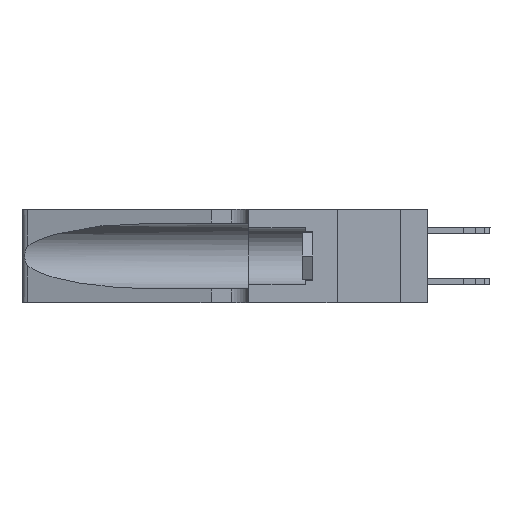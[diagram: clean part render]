
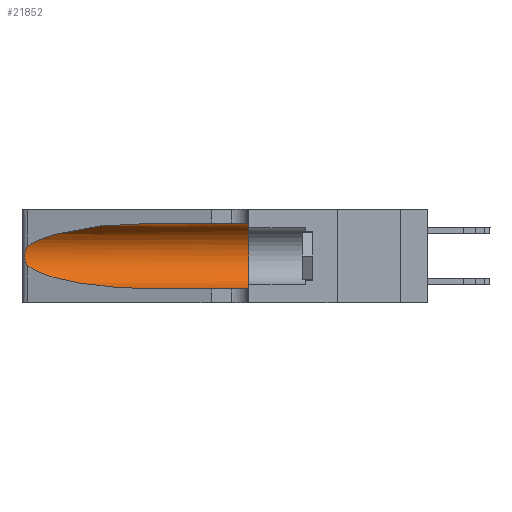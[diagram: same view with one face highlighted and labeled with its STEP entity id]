
A CAD part, left-side view. The second image highlights one B-rep face of the part: STEP entity #21852.
In plain terms, the highlighted cylindrical face has radius 3.308 mm (diameter 6.617 mm), a partial arc.
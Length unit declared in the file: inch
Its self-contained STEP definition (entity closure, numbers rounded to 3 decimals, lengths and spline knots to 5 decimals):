
#218 = CARTESIAN_POINT ( 'NONE',  ( 0.25487, 1.22718, 0.22369 ) ) ;
#322 = DIRECTION ( 'NONE',  ( 0., 0., 1. ) ) ;
#505 = ORIENTED_EDGE ( 'NONE', *, *, #8065, .T. ) ;
#927 = DIRECTION ( 'NONE',  ( 0., -1., 0. ) ) ;
#1138 = CARTESIAN_POINT ( 'NONE',  ( 0.25555, 1.22994, 0.2215 ) ) ;
#1432 = DIRECTION ( 'NONE',  ( 0., -1., 0. ) ) ;
#2477 = CARTESIAN_POINT ( 'NONE',  ( 0.18966, 0.96281, 0.05475 ) ) ;
#2498 = EDGE_CURVE ( 'NONE', #24525, #9077, #21349, .T. ) ;
#2593 = VERTEX_POINT ( 'NONE', #6418 ) ;
#2857 = CARTESIAN_POINT ( 'NONE',  ( 0.2373, 1.15595, 0.28018 ) ) ;
#3394 =( BOUNDED_CURVE ( )  B_SPLINE_CURVE ( 3, ( #6053, #19811, #2477, #18003 ),
 .UNSPECIFIED., .F., .F. ) 
 B_SPLINE_CURVE_WITH_KNOTS ( ( 4, 4 ),
 ( 3.44316, 4.71239 ),
 .UNSPECIFIED. ) 
 CURVE ( )  GEOMETRIC_REPRESENTATION_ITEM ( )  RATIONAL_B_SPLINE_CURVE ( ( 1., 0.87, 0.87, 1. ) ) 
 REPRESENTATION_ITEM ( '' )  );
#4266 = DIRECTION ( 'NONE',  ( 0., 1., 0. ) ) ;
#4814 = AXIS2_PLACEMENT_3D ( 'NONE', #12839, #927, #20414 ) ;
#5615 = VECTOR ( 'NONE', #7213, 39.37008 ) ;
#5803 = AXIS2_PLACEMENT_3D ( 'NONE', #10124, #4266, #322 ) ;
#6053 = CARTESIAN_POINT ( 'NONE',  ( 0.25487, 1.22718, 0.14631 ) ) ;
#6418 = CARTESIAN_POINT ( 'NONE',  ( 0.1305, 0.35, 0.05475 ) ) ;
#6606 = CARTESIAN_POINT ( 'NONE',  ( 0.18966, 0.96281, 0.31525 ) ) ;
#7213 = DIRECTION ( 'NONE',  ( 0., -1., 0. ) ) ;
#7472 = EDGE_CURVE ( 'NONE', #9077, #15238, #3394, .T. ) ;
#7488 = VECTOR ( 'NONE', #1432, 39.37008 ) ;
#7830 = ORIENTED_EDGE ( 'NONE', *, *, #25051, .T. ) ;
#8065 = EDGE_CURVE ( 'NONE', #15238, #2593, #12959, .T. ) ;
#8138 = CARTESIAN_POINT ( 'NONE',  ( 0.25789, 1.23486, 0.15765 ) ) ;
#9077 = VERTEX_POINT ( 'NONE', #18636 ) ;
#9919 = LINE ( 'NONE', #22778, #5615 ) ;
#10124 = CARTESIAN_POINT ( 'NONE',  ( 0.1305, 0.35, 0.185 ) ) ;
#10377 = CARTESIAN_POINT ( 'NONE',  ( 0.25555, 1.22993, 0.14849 ) ) ;
#10506 = ORIENTED_EDGE ( 'NONE', *, *, #2498, .T. ) ;
#10740 = VERTEX_POINT ( 'NONE', #15185 ) ;
#10798 = CIRCLE ( 'NONE', #5803, 0.13025 ) ;
#11205 = ORIENTED_EDGE ( 'NONE', *, *, #14524, .F. ) ;
#12324 = CARTESIAN_POINT ( 'NONE',  ( 0.26075, 1.23896, 0.19203 ) ) ;
#12839 = CARTESIAN_POINT ( 'NONE',  ( 0.1305, 1.61858, 0.185 ) ) ;
#12959 = LINE ( 'NONE', #21079, #7488 ) ;
#14297 = CARTESIAN_POINT ( 'NONE',  ( 0.25856, 1.23593, 0.16098 ) ) ;
#14524 = EDGE_CURVE ( 'NONE', #21056, #10740, #9919, .T. ) ;
#15185 = CARTESIAN_POINT ( 'NONE',  ( 0.1305, 0.35, 0.31525 ) ) ;
#15238 = VERTEX_POINT ( 'NONE', #23779 ) ;
#15631 = ORIENTED_EDGE ( 'NONE', *, *, #21116, .F. ) ;
#16015 = CARTESIAN_POINT ( 'NONE',  ( 0.25639, 1.23186, 0.15144 ) ) ;
#16291 = CARTESIAN_POINT ( 'NONE',  ( 0.25487, 1.22718, 0.14631 ) ) ;
#16509 = CARTESIAN_POINT ( 'NONE',  ( 0.25487, 1.22718, 0.22369 ) ) ;
#17447 = CARTESIAN_POINT ( 'NONE',  ( 0.25639, 1.23184, 0.21858 ) ) ;
#18003 = CARTESIAN_POINT ( 'NONE',  ( 0.1305, 0.72297, 0.05475 ) ) ;
#18119 = CARTESIAN_POINT ( 'NONE',  ( 0.26017, 1.23833, 0.17102 ) ) ;
#18145 = ORIENTED_EDGE ( 'NONE', *, *, #7472, .T. ) ;
#18294 = CARTESIAN_POINT ( 'NONE',  ( 0.26075, 1.23896, 0.178 ) ) ;
#18487 = CARTESIAN_POINT ( 'NONE',  ( 0.1305, 0.72297, 0.31525 ) ) ;
#18636 = CARTESIAN_POINT ( 'NONE',  ( 0.25487, 1.22718, 0.14631 ) ) ;
#19434 = CARTESIAN_POINT ( 'NONE',  ( 0.1305, 0.72297, 0.31525 ) ) ;
#19554 = CYLINDRICAL_SURFACE ( 'NONE', #4814, 0.13025 ) ;
#19811 = CARTESIAN_POINT ( 'NONE',  ( 0.2373, 1.15595, 0.08982 ) ) ;
#20170 = CARTESIAN_POINT ( 'NONE',  ( 0.26018, 1.23835, 0.19895 ) ) ;
#20414 = DIRECTION ( 'NONE',  ( 0., 0., -1. ) ) ;
#21056 = VERTEX_POINT ( 'NONE', #19434 ) ;
#21079 = CARTESIAN_POINT ( 'NONE',  ( 0.1305, 1.61858, 0.05475 ) ) ;
#21116 = EDGE_CURVE ( 'NONE', #10740, #2593, #10798, .T. ) ;
#21349 = B_SPLINE_CURVE_WITH_KNOTS ( 'NONE', 3,
 ( #218, #1138, #17447, #22892, #22146, #20170, #12324, #18294, #18119, #14297, #8138, #16015, #10377, #16291 ),
 .UNSPECIFIED., .F., .F.,
 ( 4, 2, 2, 2, 2, 2, 4 ),
 ( 0., 0.00027, 0.00053, 0.00107, 0.0016, 0.00187, 0.00214 ),
 .UNSPECIFIED. ) ;
#21852 = ADVANCED_FACE ( 'NONE', ( #24759 ), #19554, .F. ) ;
#22146 = CARTESIAN_POINT ( 'NONE',  ( 0.25854, 1.2359, 0.20912 ) ) ;
#22179 = EDGE_LOOP ( 'NONE', ( #7830, #10506, #18145, #505, #15631, #11205 ) ) ;
#22778 = CARTESIAN_POINT ( 'NONE',  ( 0.1305, 1.61858, 0.31525 ) ) ;
#22892 = CARTESIAN_POINT ( 'NONE',  ( 0.25787, 1.23484, 0.2124 ) ) ;
#23779 = CARTESIAN_POINT ( 'NONE',  ( 0.1305, 0.72297, 0.05475 ) ) ;
#24241 = CARTESIAN_POINT ( 'NONE',  ( 0.25487, 1.22718, 0.22369 ) ) ;
#24525 = VERTEX_POINT ( 'NONE', #16509 ) ;
#24759 = FACE_OUTER_BOUND ( 'NONE', #22179, .T. ) ;
#25051 = EDGE_CURVE ( 'NONE', #21056, #24525, #25117, .T. ) ;
#25117 =( BOUNDED_CURVE ( )  B_SPLINE_CURVE ( 3, ( #18487, #6606, #2857, #24241 ),
 .UNSPECIFIED., .F., .F. ) 
 B_SPLINE_CURVE_WITH_KNOTS ( ( 4, 4 ),
 ( 1.5708, 2.84003 ),
 .UNSPECIFIED. ) 
 CURVE ( )  GEOMETRIC_REPRESENTATION_ITEM ( )  RATIONAL_B_SPLINE_CURVE ( ( 1., 0.87, 0.87, 1. ) ) 
 REPRESENTATION_ITEM ( '' )  );
